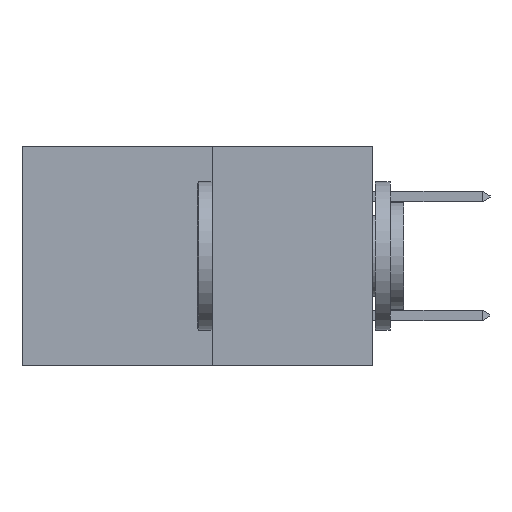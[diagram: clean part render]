
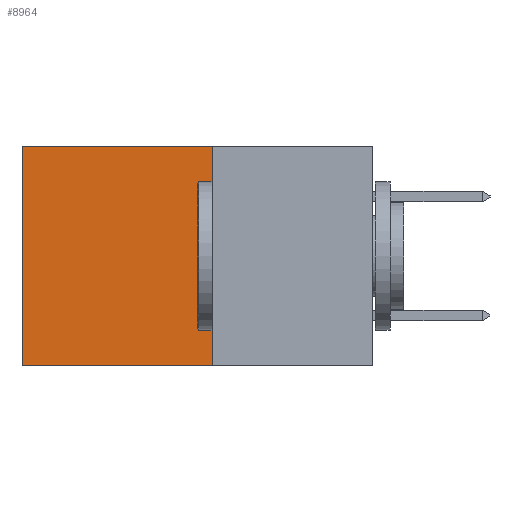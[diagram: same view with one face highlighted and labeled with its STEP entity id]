
A CAD part, left-side view. The second image highlights one B-rep face of the part: STEP entity #8964.
In plain terms, the highlighted planar face has unit normal (-1, 0, 0).
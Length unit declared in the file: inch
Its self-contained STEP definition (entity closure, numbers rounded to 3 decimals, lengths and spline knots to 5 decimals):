
#115 = DIRECTION ( 'NONE',  ( 0., 0., -1. ) ) ;
#313 = CARTESIAN_POINT ( 'NONE',  ( 0.277, 0.59, 0. ) ) ;
#591 = ORIENTED_EDGE ( 'NONE', *, *, #18741, .T. ) ;
#2471 = CARTESIAN_POINT ( 'NONE',  ( 0.277, 0.27, 0. ) ) ;
#2490 = DIRECTION ( 'NONE',  ( 0., 1., 0. ) ) ;
#2748 = EDGE_CURVE ( 'NONE', #12715, #13216, #19413, .T. ) ;
#3543 = CARTESIAN_POINT ( 'NONE',  ( 0.277, 0.27, -0.37 ) ) ;
#3704 = VECTOR ( 'NONE', #6840, 39.37008 ) ;
#4230 = CARTESIAN_POINT ( 'NONE',  ( 0.277, 0.27, -0.37 ) ) ;
#4478 = VECTOR ( 'NONE', #14375, 39.37008 ) ;
#4920 = VERTEX_POINT ( 'NONE', #313 ) ;
#5763 = DIRECTION ( 'NONE',  ( 0., 0., -1. ) ) ;
#6266 = EDGE_CURVE ( 'NONE', #13216, #15461, #19038, .T. ) ;
#6840 = DIRECTION ( 'NONE',  ( 0., 1., 0. ) ) ;
#7026 = EDGE_CURVE ( 'NONE', #12715, #4920, #10043, .T. ) ;
#8120 = FACE_OUTER_BOUND ( 'NONE', #9400, .T. ) ;
#8138 = VECTOR ( 'NONE', #115, 39.37008 ) ;
#8964 = ADVANCED_FACE ( 'NONE', ( #8120 ), #13109, .F. ) ;
#9400 = EDGE_LOOP ( 'NONE', ( #591, #13136, #17540, #10186 ) ) ;
#10043 = LINE ( 'NONE', #2471, #17397 ) ;
#10186 = ORIENTED_EDGE ( 'NONE', *, *, #7026, .T. ) ;
#10716 = CARTESIAN_POINT ( 'NONE',  ( 0.277, 0.59, -0.37 ) ) ;
#10755 = CARTESIAN_POINT ( 'NONE',  ( 0.277, 0.27, -0.37 ) ) ;
#10859 = CARTESIAN_POINT ( 'NONE',  ( 0.277, 0.27, 0. ) ) ;
#12152 = AXIS2_PLACEMENT_3D ( 'NONE', #4230, #14578, #5763 ) ;
#12715 = VERTEX_POINT ( 'NONE', #10859 ) ;
#12820 = LINE ( 'NONE', #12908, #4478 ) ;
#12908 = CARTESIAN_POINT ( 'NONE',  ( 0.277, 0.59, -0.37 ) ) ;
#13109 = PLANE ( 'NONE',  #12152 ) ;
#13136 = ORIENTED_EDGE ( 'NONE', *, *, #6266, .F. ) ;
#13216 = VERTEX_POINT ( 'NONE', #19322 ) ;
#14375 = DIRECTION ( 'NONE',  ( 0., 0., -1. ) ) ;
#14578 = DIRECTION ( 'NONE',  ( 1., 0., 0. ) ) ;
#15461 = VERTEX_POINT ( 'NONE', #10716 ) ;
#17397 = VECTOR ( 'NONE', #2490, 39.37008 ) ;
#17540 = ORIENTED_EDGE ( 'NONE', *, *, #2748, .F. ) ;
#18741 = EDGE_CURVE ( 'NONE', #4920, #15461, #12820, .T. ) ;
#19038 = LINE ( 'NONE', #3543, #3704 ) ;
#19322 = CARTESIAN_POINT ( 'NONE',  ( 0.277, 0.27, -0.37 ) ) ;
#19413 = LINE ( 'NONE', #10755, #8138 ) ;
